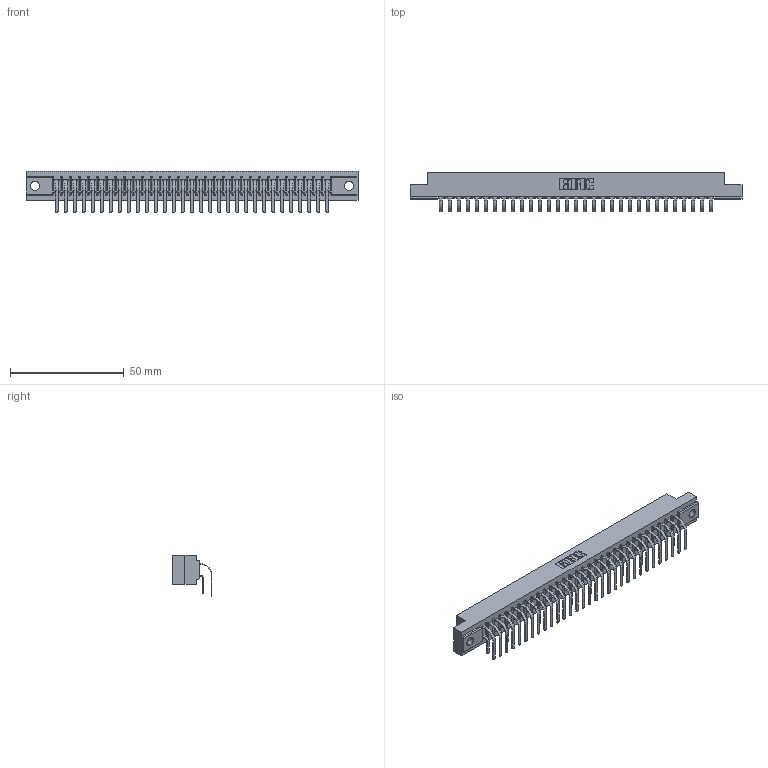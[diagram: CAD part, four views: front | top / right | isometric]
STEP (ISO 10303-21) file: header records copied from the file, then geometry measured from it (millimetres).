
FILE_DESCRIPTION (( 'STEP AP203' ), '1' );
FILE_NAME ('357-062-559-202.STEP', '2022-07-08T21:43:54', ( '' ), ( '' ), 'SwSTEP 2.0', 'SolidWorks 2020', '' );
FILE_SCHEMA (( 'CONFIG_CONTROL_DESIGN' ));
Length unit declared in the file: inch
Products named in the file (4): 307 Part_.128 Dia Mounting Holes; 357-062-559-202; 307-290-001_559 - 2 (Single); 307-290-001_558 559 - 1 (Single)
Assembly tree (63 placements, depth 2):
  357-062-559-202
    307 Part_.128 Dia Mounting Holes
    307-290-001_558 559 - 1 (Single)  x31
    307-290-001_559 - 2 (Single)  x31
Bounding box: 145.85 x 17.51 x 18.07 mm (x, y, z)
Volume: 15576.5 mm3; surface area: 19966.8 mm2
Topology: 63 solids, 63 shells, 3250 faces, 9127 edges, 5914 vertices
Faces by surface type: plane 2116, cylinder 1070, sphere 64
Entity records: 30373 total; most frequent: CARTESIAN_POINT 4973, ORIENTED_EDGE 4926, DIRECTION 4875, EDGE_CURVE 2463, VECTOR 1883, LINE 1883, VERTEX_POINT 1594, AXIS2_PLACEMENT_3D 1496
